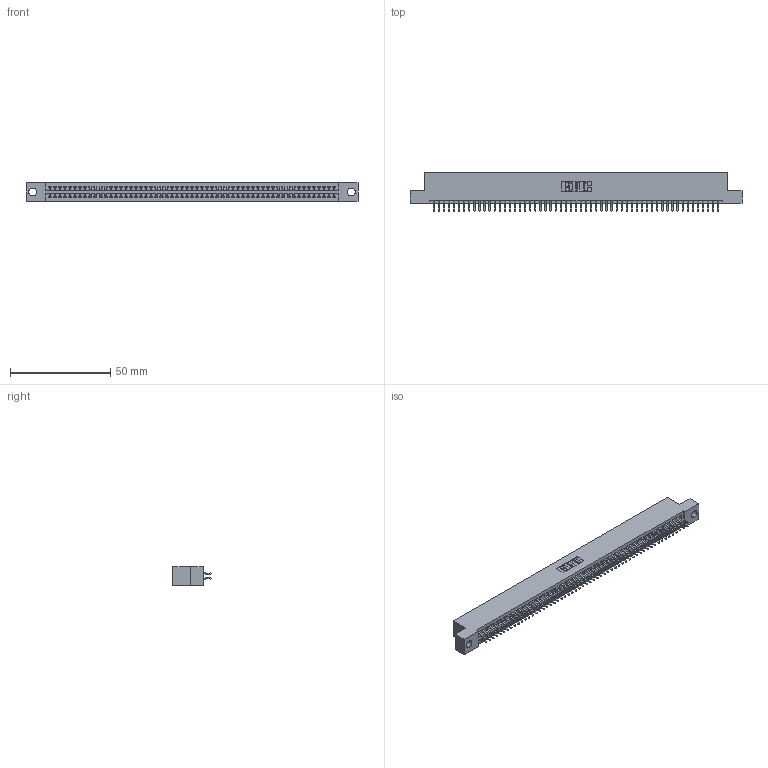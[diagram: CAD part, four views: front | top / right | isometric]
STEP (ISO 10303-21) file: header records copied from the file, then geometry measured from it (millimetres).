
FILE_DESCRIPTION (( 'STEP AP203' ), '1' );
FILE_NAME ('395-114-556-204.STEP', '2018-12-01T18:30:35', ( '' ), ( '' ), 'SwSTEP 2.0', 'SolidWorks 2016', '' );
FILE_SCHEMA (( 'CONFIG_CONTROL_DESIGN' ));
Length unit declared in the file: inch
Products named in the file (3): 395-114-556-204; 345 Part_Flush Mounting Lugs - 0.156 Dia-TH; 345-292-001_556 Tail
Assembly tree (115 placements, depth 2):
  395-114-556-204
    345 Part_Flush Mounting Lugs - 0.156 Dia-TH
    345-292-001_556 Tail  x114
Bounding box: 165.99 x 19.24 x 9.4 mm (x, y, z)
Volume: 16171.2 mm3; surface area: 23909.7 mm2
Topology: 115 solids, 115 shells, 6510 faces, 19379 edges, 12766 vertices
Faces by surface type: plane 4298, cylinder 2212
Entity records: 42927 total; most frequent: CARTESIAN_POINT 7196, ORIENTED_EDGE 7118, DIRECTION 6315, EDGE_CURVE 3559, VECTOR 3191, LINE 3191, VERTEX_POINT 2370, AXIS2_PLACEMENT_3D 1562
